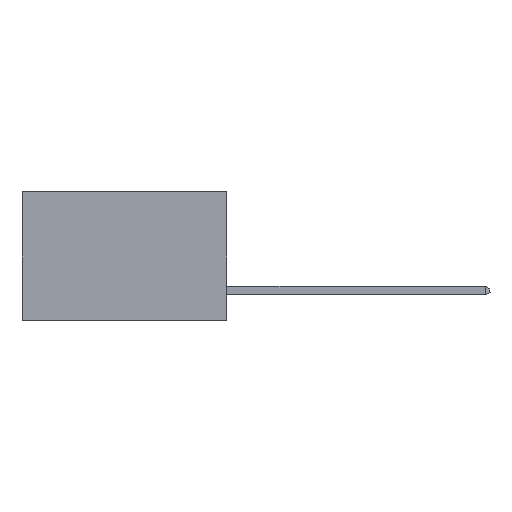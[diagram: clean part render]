
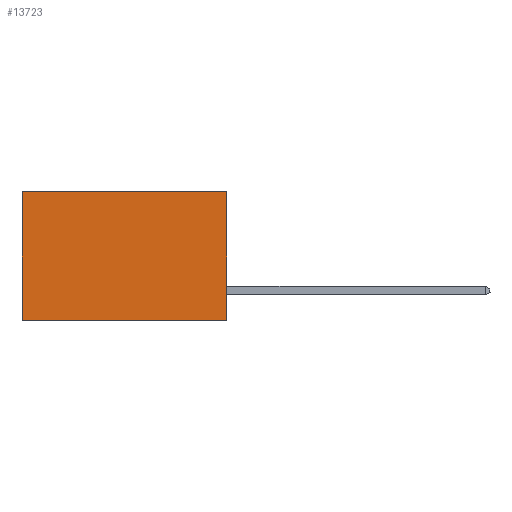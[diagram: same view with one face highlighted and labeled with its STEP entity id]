
A CAD part, left-side view. The second image highlights one B-rep face of the part: STEP entity #13723.
In plain terms, the highlighted planar face has unit normal (-1, 0, 0).
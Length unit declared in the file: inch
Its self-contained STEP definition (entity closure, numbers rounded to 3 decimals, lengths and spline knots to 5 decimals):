
#566 = LINE ( 'NONE', #26329, #16736 ) ;
#1315 = DIRECTION ( 'NONE',  ( 0., 1., 0. ) ) ;
#1351 = EDGE_CURVE ( 'NONE', #14280, #1560, #10126, .T. ) ;
#1441 = CARTESIAN_POINT ( 'NONE',  ( 0.277, 0., 0. ) ) ;
#1560 = VERTEX_POINT ( 'NONE', #26325 ) ;
#2577 = DIRECTION ( 'NONE',  ( 0., 1., 0. ) ) ;
#5104 = CARTESIAN_POINT ( 'NONE',  ( 0.277, 0.59, 0. ) ) ;
#6107 = CARTESIAN_POINT ( 'NONE',  ( 0.277, 0., -0.37 ) ) ;
#6472 = ORIENTED_EDGE ( 'NONE', *, *, #12556, .T. ) ;
#7912 = VERTEX_POINT ( 'NONE', #5104 ) ;
#8261 = PLANE ( 'NONE',  #18860 ) ;
#8463 = EDGE_CURVE ( 'NONE', #14280, #7912, #21909, .T. ) ;
#8883 = ORIENTED_EDGE ( 'NONE', *, *, #22699, .F. ) ;
#9054 = EDGE_LOOP ( 'NONE', ( #6472, #8883, #16182, #14250 ) ) ;
#10126 = LINE ( 'NONE', #16357, #19960 ) ;
#10372 = DIRECTION ( 'NONE',  ( 1., 0., 0. ) ) ;
#12556 = EDGE_CURVE ( 'NONE', #7912, #19799, #26033, .T. ) ;
#13723 = ADVANCED_FACE ( 'NONE', ( #18919 ), #8261, .F. ) ;
#14250 = ORIENTED_EDGE ( 'NONE', *, *, #8463, .T. ) ;
#14280 = VERTEX_POINT ( 'NONE', #18407 ) ;
#16182 = ORIENTED_EDGE ( 'NONE', *, *, #1351, .F. ) ;
#16357 = CARTESIAN_POINT ( 'NONE',  ( 0.277, 0., -0.37 ) ) ;
#16709 = DIRECTION ( 'NONE',  ( 0., 0., -1. ) ) ;
#16736 = VECTOR ( 'NONE', #1315, 39.37008 ) ;
#16784 = CARTESIAN_POINT ( 'NONE',  ( 0.277, 0.59, -0.37 ) ) ;
#18407 = CARTESIAN_POINT ( 'NONE',  ( 0.277, 0., 0. ) ) ;
#18860 = AXIS2_PLACEMENT_3D ( 'NONE', #6107, #10372, #24919 ) ;
#18919 = FACE_OUTER_BOUND ( 'NONE', #9054, .T. ) ;
#19144 = CARTESIAN_POINT ( 'NONE',  ( 0.277, 0.59, -0.37 ) ) ;
#19799 = VERTEX_POINT ( 'NONE', #19144 ) ;
#19960 = VECTOR ( 'NONE', #16709, 39.37008 ) ;
#21256 = VECTOR ( 'NONE', #26985, 39.37008 ) ;
#21909 = LINE ( 'NONE', #1441, #27008 ) ;
#22699 = EDGE_CURVE ( 'NONE', #1560, #19799, #566, .T. ) ;
#24919 = DIRECTION ( 'NONE',  ( 0., 0., -1. ) ) ;
#26033 = LINE ( 'NONE', #16784, #21256 ) ;
#26325 = CARTESIAN_POINT ( 'NONE',  ( 0.277, 0., -0.37 ) ) ;
#26329 = CARTESIAN_POINT ( 'NONE',  ( 0.277, 0., -0.37 ) ) ;
#26985 = DIRECTION ( 'NONE',  ( 0., 0., -1. ) ) ;
#27008 = VECTOR ( 'NONE', #2577, 39.37008 ) ;
